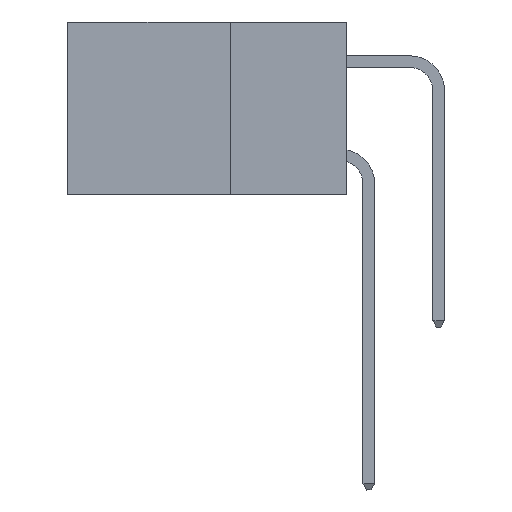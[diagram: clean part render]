
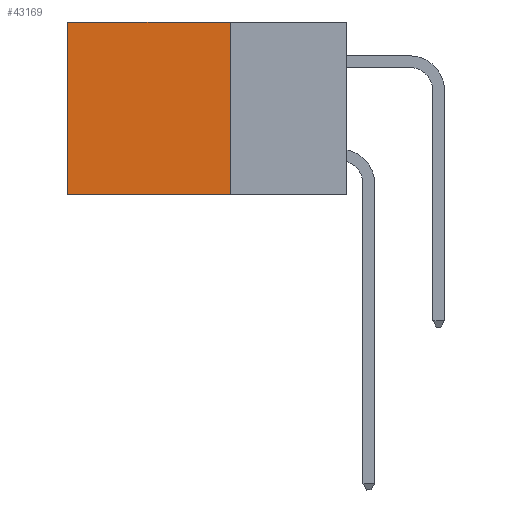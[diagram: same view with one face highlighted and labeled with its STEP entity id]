
A CAD part, left-side view. The second image highlights one B-rep face of the part: STEP entity #43169.
In plain terms, the highlighted planar face has unit normal (-1, 0, 0).
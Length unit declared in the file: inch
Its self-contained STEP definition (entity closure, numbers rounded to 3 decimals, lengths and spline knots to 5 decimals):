
#167 = LINE ( 'NONE', #44618, #15175 ) ;
#351 = VECTOR ( 'NONE', #38713, 39.37008 ) ;
#1378 = LINE ( 'NONE', #34084, #46400 ) ;
#4860 = ORIENTED_EDGE ( 'NONE', *, *, #37348, .T. ) ;
#5977 = VERTEX_POINT ( 'NONE', #46925 ) ;
#8042 = VERTEX_POINT ( 'NONE', #18692 ) ;
#8710 = LINE ( 'NONE', #13334, #41419 ) ;
#8905 = ORIENTED_EDGE ( 'NONE', *, *, #48858, .T. ) ;
#11192 = FACE_OUTER_BOUND ( 'NONE', #46673, .T. ) ;
#11445 = LINE ( 'NONE', #43307, #351 ) ;
#13334 = CARTESIAN_POINT ( 'NONE',  ( 0.2875, 0.25, -0.37 ) ) ;
#13509 = DIRECTION ( 'NONE',  ( 0., 1., 0. ) ) ;
#15175 = VECTOR ( 'NONE', #32343, 39.37008 ) ;
#17158 = PLANE ( 'NONE',  #37636 ) ;
#17501 = DIRECTION ( 'NONE',  ( 0., 1., 0. ) ) ;
#18692 = CARTESIAN_POINT ( 'NONE',  ( 0.2875, 0.25, 0. ) ) ;
#23036 = EDGE_CURVE ( 'NONE', #8042, #37243, #11445, .T. ) ;
#24834 = CARTESIAN_POINT ( 'NONE',  ( 0.2875, 0.25, -0.37 ) ) ;
#29171 = CARTESIAN_POINT ( 'NONE',  ( 0.2875, 0.25, 0. ) ) ;
#30300 = CARTESIAN_POINT ( 'NONE',  ( 0.2875, 0.6, 0. ) ) ;
#32343 = DIRECTION ( 'NONE',  ( 0., 0., -1. ) ) ;
#34084 = CARTESIAN_POINT ( 'NONE',  ( 0.2875, 0.25, 0. ) ) ;
#37243 = VERTEX_POINT ( 'NONE', #24834 ) ;
#37348 = EDGE_CURVE ( 'NONE', #8042, #49159, #1378, .T. ) ;
#37636 = AXIS2_PLACEMENT_3D ( 'NONE', #29171, #41974, #54018 ) ;
#38713 = DIRECTION ( 'NONE',  ( 0., 0., -1. ) ) ;
#41372 = EDGE_CURVE ( 'NONE', #37243, #5977, #8710, .T. ) ;
#41419 = VECTOR ( 'NONE', #17501, 39.37008 ) ;
#41974 = DIRECTION ( 'NONE',  ( 1., 0., 0. ) ) ;
#43169 = ADVANCED_FACE ( 'NONE', ( #11192 ), #17158, .F. ) ;
#43307 = CARTESIAN_POINT ( 'NONE',  ( 0.2875, 0.25, 0. ) ) ;
#44618 = CARTESIAN_POINT ( 'NONE',  ( 0.2875, 0.6, 0. ) ) ;
#46400 = VECTOR ( 'NONE', #13509, 39.37008 ) ;
#46673 = EDGE_LOOP ( 'NONE', ( #8905, #53604, #49634, #4860 ) ) ;
#46925 = CARTESIAN_POINT ( 'NONE',  ( 0.2875, 0.6, -0.37 ) ) ;
#48858 = EDGE_CURVE ( 'NONE', #49159, #5977, #167, .T. ) ;
#49159 = VERTEX_POINT ( 'NONE', #30300 ) ;
#49634 = ORIENTED_EDGE ( 'NONE', *, *, #23036, .F. ) ;
#53604 = ORIENTED_EDGE ( 'NONE', *, *, #41372, .F. ) ;
#54018 = DIRECTION ( 'NONE',  ( 0., 0., -1. ) ) ;
